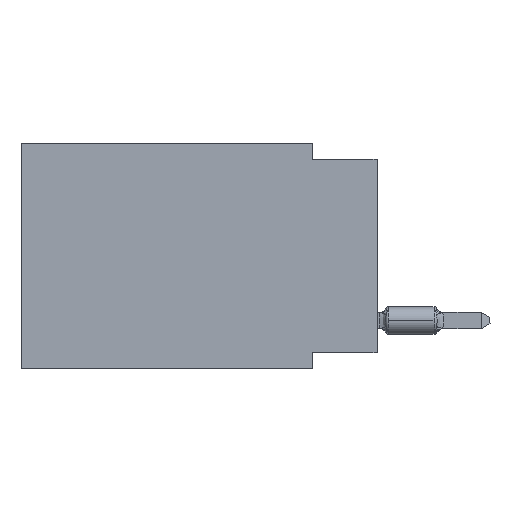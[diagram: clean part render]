
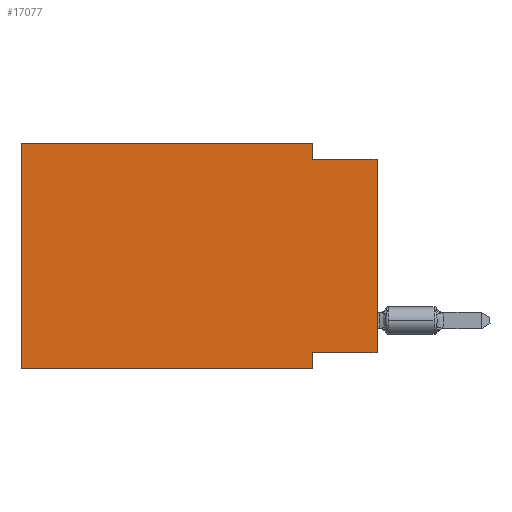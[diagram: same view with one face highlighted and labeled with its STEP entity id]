
A CAD part, left-side view. The second image highlights one B-rep face of the part: STEP entity #17077.
In plain terms, the highlighted planar face has unit normal (-1, 0, 0).
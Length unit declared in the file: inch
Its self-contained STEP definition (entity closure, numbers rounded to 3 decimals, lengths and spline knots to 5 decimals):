
#203 = DIRECTION ( 'NONE',  ( 0., -1., 0. ) ) ;
#368 = CARTESIAN_POINT ( 'NONE',  ( 0., 0.55, -0.35 ) ) ;
#665 = VERTEX_POINT ( 'NONE', #11460 ) ;
#838 = EDGE_CURVE ( 'NONE', #9658, #8423, #14376, .T. ) ;
#1123 = VERTEX_POINT ( 'NONE', #2293 ) ;
#1142 = ORIENTED_EDGE ( 'NONE', *, *, #838, .T. ) ;
#1754 = VECTOR ( 'NONE', #9919, 39.37008 ) ;
#1795 = ORIENTED_EDGE ( 'NONE', *, *, #7815, .F. ) ;
#1810 = CARTESIAN_POINT ( 'NONE',  ( 0., 0.55, 0. ) ) ;
#1944 = VECTOR ( 'NONE', #12769, 39.37008 ) ;
#2042 = LINE ( 'NONE', #10564, #12592 ) ;
#2293 = CARTESIAN_POINT ( 'NONE',  ( 0., 0.1, 0. ) ) ;
#2440 = VERTEX_POINT ( 'NONE', #12324 ) ;
#3163 = EDGE_CURVE ( 'NONE', #1123, #7624, #16551, .T. ) ;
#3204 = CARTESIAN_POINT ( 'NONE',  ( 0., 0.1, -0.325 ) ) ;
#4076 = CARTESIAN_POINT ( 'NONE',  ( 0., 0., -0.325 ) ) ;
#4112 = EDGE_CURVE ( 'NONE', #17365, #8423, #16727, .T. ) ;
#4302 = CARTESIAN_POINT ( 'NONE',  ( 0., 0.1, 0. ) ) ;
#4751 = VECTOR ( 'NONE', #16663, 39.37008 ) ;
#5778 = VECTOR ( 'NONE', #9456, 39.37008 ) ;
#7109 = CARTESIAN_POINT ( 'NONE',  ( 0., 0.55, -0.35 ) ) ;
#7386 = EDGE_LOOP ( 'NONE', ( #9327, #15307, #8877, #1795, #10070, #1142, #8127, #10667 ) ) ;
#7624 = VERTEX_POINT ( 'NONE', #12974 ) ;
#7815 = EDGE_CURVE ( 'NONE', #665, #1123, #8938, .T. ) ;
#7994 = DIRECTION ( 'NONE',  ( 1., 0., 0. ) ) ;
#8127 = ORIENTED_EDGE ( 'NONE', *, *, #4112, .F. ) ;
#8423 = VERTEX_POINT ( 'NONE', #12237 ) ;
#8472 = EDGE_CURVE ( 'NONE', #7624, #2440, #15973, .T. ) ;
#8877 = ORIENTED_EDGE ( 'NONE', *, *, #3163, .F. ) ;
#8938 = LINE ( 'NONE', #12029, #15786 ) ;
#9327 = ORIENTED_EDGE ( 'NONE', *, *, #11371, .T. ) ;
#9456 = DIRECTION ( 'NONE',  ( 0., 0., -1. ) ) ;
#9658 = VERTEX_POINT ( 'NONE', #368 ) ;
#9919 = DIRECTION ( 'NONE',  ( 0., -1., 0. ) ) ;
#10014 = VERTEX_POINT ( 'NONE', #4076 ) ;
#10070 = ORIENTED_EDGE ( 'NONE', *, *, #17353, .F. ) ;
#10564 = CARTESIAN_POINT ( 'NONE',  ( 0., 0., 0. ) ) ;
#10660 = DIRECTION ( 'NONE',  ( 0., -1., 0. ) ) ;
#10667 = ORIENTED_EDGE ( 'NONE', *, *, #13943, .F. ) ;
#10721 = PLANE ( 'NONE',  #14995 ) ;
#10768 = DIRECTION ( 'NONE',  ( 0., 1., 0. ) ) ;
#11284 = CARTESIAN_POINT ( 'NONE',  ( 0., 0., -0.025 ) ) ;
#11371 = EDGE_CURVE ( 'NONE', #10014, #2440, #2042, .T. ) ;
#11460 = CARTESIAN_POINT ( 'NONE',  ( 0., 0.55, 0. ) ) ;
#11889 = LINE ( 'NONE', #12015, #14657 ) ;
#12015 = CARTESIAN_POINT ( 'NONE',  ( 0., 0., -0.325 ) ) ;
#12029 = CARTESIAN_POINT ( 'NONE',  ( 0., 0.55, 0. ) ) ;
#12237 = CARTESIAN_POINT ( 'NONE',  ( 0., 0.1, -0.35 ) ) ;
#12324 = CARTESIAN_POINT ( 'NONE',  ( 0., 0., -0.025 ) ) ;
#12592 = VECTOR ( 'NONE', #13298, 39.37008 ) ;
#12769 = DIRECTION ( 'NONE',  ( 0., 0., 1. ) ) ;
#12974 = CARTESIAN_POINT ( 'NONE',  ( 0., 0.1, -0.025 ) ) ;
#13298 = DIRECTION ( 'NONE',  ( 0., 0., 1. ) ) ;
#13943 = EDGE_CURVE ( 'NONE', #10014, #17365, #11889, .T. ) ;
#14376 = LINE ( 'NONE', #7109, #17593 ) ;
#14657 = VECTOR ( 'NONE', #10768, 39.37008 ) ;
#14859 = CARTESIAN_POINT ( 'NONE',  ( 0., 0.1, -0.35 ) ) ;
#14995 = AXIS2_PLACEMENT_3D ( 'NONE', #16204, #7994, #17579 ) ;
#15307 = ORIENTED_EDGE ( 'NONE', *, *, #8472, .F. ) ;
#15786 = VECTOR ( 'NONE', #10660, 39.37008 ) ;
#15973 = LINE ( 'NONE', #11284, #1754 ) ;
#16204 = CARTESIAN_POINT ( 'NONE',  ( 0., 0.55, 0. ) ) ;
#16551 = LINE ( 'NONE', #4302, #4751 ) ;
#16565 = LINE ( 'NONE', #1810, #1944 ) ;
#16663 = DIRECTION ( 'NONE',  ( 0., 0., -1. ) ) ;
#16727 = LINE ( 'NONE', #14859, #5778 ) ;
#17077 = ADVANCED_FACE ( 'NONE', ( #17226 ), #10721, .F. ) ;
#17226 = FACE_OUTER_BOUND ( 'NONE', #7386, .T. ) ;
#17353 = EDGE_CURVE ( 'NONE', #9658, #665, #16565, .T. ) ;
#17365 = VERTEX_POINT ( 'NONE', #3204 ) ;
#17579 = DIRECTION ( 'NONE',  ( 0., 0., -1. ) ) ;
#17593 = VECTOR ( 'NONE', #203, 39.37008 ) ;
